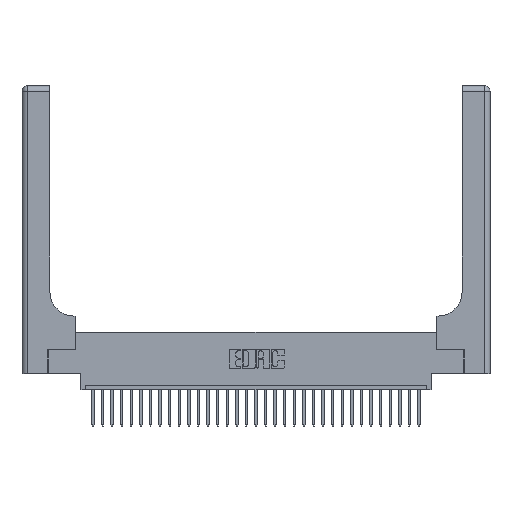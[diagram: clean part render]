
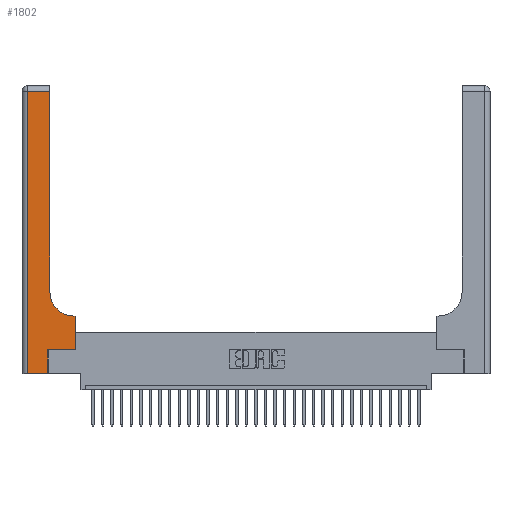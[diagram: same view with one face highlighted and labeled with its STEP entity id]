
A CAD part, top view. The second image highlights one B-rep face of the part: STEP entity #1802.
In plain terms, the highlighted planar face has unit normal (0, 0, 1).
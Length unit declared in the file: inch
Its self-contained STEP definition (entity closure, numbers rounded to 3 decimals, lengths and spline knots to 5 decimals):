
#72 = VERTEX_POINT ( 'NONE', #16608 ) ;
#142 = VECTOR ( 'NONE', #19762, 39.37008 ) ;
#306 = EDGE_CURVE ( 'NONE', #32587, #25492, #20205, .T. ) ;
#1372 = VERTEX_POINT ( 'NONE', #27390 ) ;
#1802 = ADVANCED_FACE ( 'NONE', ( #21682 ), #17291, .F. ) ;
#2752 = DIRECTION ( 'NONE',  ( -1., 0., 0. ) ) ;
#2757 = CARTESIAN_POINT ( 'NONE',  ( 0.2915, 3., 0.37 ) ) ;
#2933 = EDGE_CURVE ( 'NONE', #19307, #16103, #30280, .T. ) ;
#3813 = LINE ( 'NONE', #22806, #24624 ) ;
#4378 = VECTOR ( 'NONE', #15507, 39.37008 ) ;
#4464 = ORIENTED_EDGE ( 'NONE', *, *, #306, .T. ) ;
#4849 = LINE ( 'NONE', #7021, #142 ) ;
#5742 = CARTESIAN_POINT ( 'NONE',  ( 0.06, 2.94, 0.37 ) ) ;
#5879 = EDGE_LOOP ( 'NONE', ( #4464, #20100, #28466, #19231, #10244, #9048, #19398, #16988, #8372 ) ) ;
#6842 = VECTOR ( 'NONE', #12309, 39.37008 ) ;
#6854 = DIRECTION ( 'NONE',  ( 0., 0., -1. ) ) ;
#7021 = CARTESIAN_POINT ( 'NONE',  ( 0.5585, 0.25, 0.37 ) ) ;
#7029 = CARTESIAN_POINT ( 'NONE',  ( 0.5585, 0.6, 0.37 ) ) ;
#8372 = ORIENTED_EDGE ( 'NONE', *, *, #27765, .T. ) ;
#8379 = VERTEX_POINT ( 'NONE', #7029 ) ;
#9048 = ORIENTED_EDGE ( 'NONE', *, *, #2933, .T. ) ;
#10013 = CARTESIAN_POINT ( 'NONE',  ( 0., 0., 0.37 ) ) ;
#10142 = CARTESIAN_POINT ( 'NONE',  ( 0.2915, 0.85, 0.37 ) ) ;
#10225 = DIRECTION ( 'NONE',  ( 1., 0., 0. ) ) ;
#10244 = ORIENTED_EDGE ( 'NONE', *, *, #20118, .T. ) ;
#11427 = CARTESIAN_POINT ( 'NONE',  ( 0.269, 0.25, 0.37 ) ) ;
#11940 = VECTOR ( 'NONE', #23905, 39.37008 ) ;
#12309 = DIRECTION ( 'NONE',  ( 0., 1., 0. ) ) ;
#12547 = AXIS2_PLACEMENT_3D ( 'NONE', #19815, #6854, #22337 ) ;
#13656 = CARTESIAN_POINT ( 'NONE',  ( 0.2915, 2.94, 0.37 ) ) ;
#14682 = LINE ( 'NONE', #10013, #27249 ) ;
#14783 = VERTEX_POINT ( 'NONE', #5742 ) ;
#14907 = EDGE_CURVE ( 'NONE', #16103, #8379, #4849, .T. ) ;
#15079 = LINE ( 'NONE', #26428, #11940 ) ;
#15134 = CARTESIAN_POINT ( 'NONE',  ( 0.5585, 0.25, 0.37 ) ) ;
#15306 = DIRECTION ( 'NONE',  ( 0., 0., -1. ) ) ;
#15507 = DIRECTION ( 'NONE',  ( 0., -1., 0. ) ) ;
#15848 = DIRECTION ( 'NONE',  ( 1., 0., 0. ) ) ;
#16103 = VERTEX_POINT ( 'NONE', #15134 ) ;
#16451 = EDGE_CURVE ( 'NONE', #18052, #72, #14682, .T. ) ;
#16608 = CARTESIAN_POINT ( 'NONE',  ( 0.269, 0., 0.37 ) ) ;
#16988 = ORIENTED_EDGE ( 'NONE', *, *, #22225, .T. ) ;
#17291 = PLANE ( 'NONE',  #12547 ) ;
#17694 = CARTESIAN_POINT ( 'NONE',  ( 0.5415, 0.85, 0.37 ) ) ;
#18052 = VERTEX_POINT ( 'NONE', #25037 ) ;
#19231 = ORIENTED_EDGE ( 'NONE', *, *, #16451, .T. ) ;
#19264 = VECTOR ( 'NONE', #2752, 39.37008 ) ;
#19307 = VERTEX_POINT ( 'NONE', #11427 ) ;
#19398 = ORIENTED_EDGE ( 'NONE', *, *, #14907, .T. ) ;
#19762 = DIRECTION ( 'NONE',  ( 0., 1., 0. ) ) ;
#19815 = CARTESIAN_POINT ( 'NONE',  ( 0., 3., 0.37 ) ) ;
#20100 = ORIENTED_EDGE ( 'NONE', *, *, #26751, .T. ) ;
#20118 = EDGE_CURVE ( 'NONE', #72, #19307, #15079, .T. ) ;
#20205 = LINE ( 'NONE', #2757, #6842 ) ;
#20376 = DIRECTION ( 'NONE',  ( -1., 0., 0. ) ) ;
#20393 = CARTESIAN_POINT ( 'NONE',  ( 0.2915, 0.6, 0.37 ) ) ;
#20703 = EDGE_CURVE ( 'NONE', #14783, #18052, #23691, .T. ) ;
#21623 = LINE ( 'NONE', #20393, #19264 ) ;
#21682 = FACE_OUTER_BOUND ( 'NONE', #5879, .T. ) ;
#21932 = AXIS2_PLACEMENT_3D ( 'NONE', #17694, #15306, #10225 ) ;
#22225 = EDGE_CURVE ( 'NONE', #8379, #1372, #21623, .T. ) ;
#22337 = DIRECTION ( 'NONE',  ( -1., 0., 0. ) ) ;
#22806 = CARTESIAN_POINT ( 'NONE',  ( 0., 2.94, 0.37 ) ) ;
#23691 = LINE ( 'NONE', #31014, #4378 ) ;
#23905 = DIRECTION ( 'NONE',  ( 0., 1., 0. ) ) ;
#24624 = VECTOR ( 'NONE', #20376, 39.37008 ) ;
#25037 = CARTESIAN_POINT ( 'NONE',  ( 0.06, 0., 0.37 ) ) ;
#25492 = VERTEX_POINT ( 'NONE', #13656 ) ;
#26428 = CARTESIAN_POINT ( 'NONE',  ( 0.269, 0., 0.37 ) ) ;
#26751 = EDGE_CURVE ( 'NONE', #25492, #14783, #3813, .T. ) ;
#27249 = VECTOR ( 'NONE', #30383, 39.37008 ) ;
#27390 = CARTESIAN_POINT ( 'NONE',  ( 0.5415, 0.6, 0.37 ) ) ;
#27765 = EDGE_CURVE ( 'NONE', #1372, #32587, #28945, .T. ) ;
#28466 = ORIENTED_EDGE ( 'NONE', *, *, #20703, .T. ) ;
#28506 = CARTESIAN_POINT ( 'NONE',  ( 0.269, 0.25, 0.37 ) ) ;
#28727 = VECTOR ( 'NONE', #15848, 39.37008 ) ;
#28945 = CIRCLE ( 'NONE', #21932, 0.25 ) ;
#30280 = LINE ( 'NONE', #28506, #28727 ) ;
#30383 = DIRECTION ( 'NONE',  ( 1., 0., 0. ) ) ;
#31014 = CARTESIAN_POINT ( 'NONE',  ( 0.06, 3., 0.37 ) ) ;
#32587 = VERTEX_POINT ( 'NONE', #10142 ) ;
